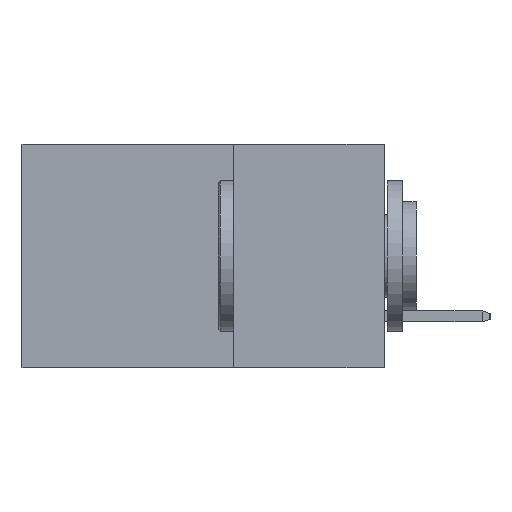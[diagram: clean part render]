
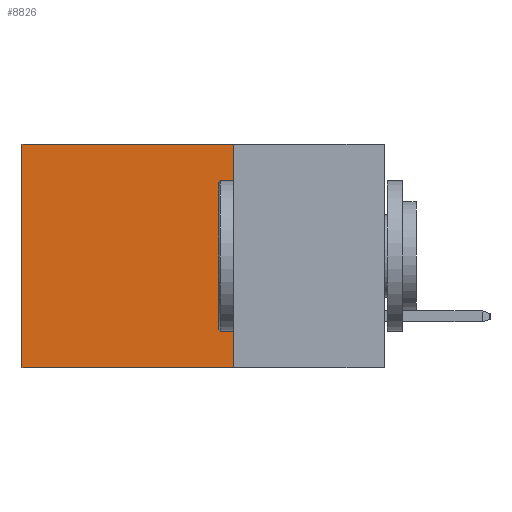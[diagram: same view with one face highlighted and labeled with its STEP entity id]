
A CAD part, left-side view. The second image highlights one B-rep face of the part: STEP entity #8826.
In plain terms, the highlighted planar face has unit normal (-1, 0, 0).
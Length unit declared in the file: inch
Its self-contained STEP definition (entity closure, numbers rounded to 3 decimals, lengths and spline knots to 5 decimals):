
#191 = DIRECTION ( 'NONE',  ( 0., 0., -1. ) ) ;
#909 = DIRECTION ( 'NONE',  ( 0., 1., 0. ) ) ;
#981 = CARTESIAN_POINT ( 'NONE',  ( 0.298, 0.25, -0.37 ) ) ;
#2281 = EDGE_CURVE ( 'NONE', #13256, #20622, #2415, .T. ) ;
#2415 = LINE ( 'NONE', #9149, #18506 ) ;
#2571 = VERTEX_POINT ( 'NONE', #17426 ) ;
#2588 = DIRECTION ( 'NONE',  ( 0., 1., 0. ) ) ;
#2706 = VECTOR ( 'NONE', #191, 39.37008 ) ;
#3196 = AXIS2_PLACEMENT_3D ( 'NONE', #12949, #9697, #21202 ) ;
#4285 = ORIENTED_EDGE ( 'NONE', *, *, #2281, .T. ) ;
#5083 = LINE ( 'NONE', #21082, #12897 ) ;
#5453 = ORIENTED_EDGE ( 'NONE', *, *, #9980, .F. ) ;
#6153 = EDGE_CURVE ( 'NONE', #2571, #19779, #18975, .T. ) ;
#6751 = CARTESIAN_POINT ( 'NONE',  ( 0.298, 0.6, 0. ) ) ;
#7078 = CARTESIAN_POINT ( 'NONE',  ( 0.298, 0.25, 0. ) ) ;
#7529 = EDGE_LOOP ( 'NONE', ( #19996, #15564, #5453, #4285 ) ) ;
#7881 = DIRECTION ( 'NONE',  ( 0., 0., -1. ) ) ;
#7948 = CARTESIAN_POINT ( 'NONE',  ( 0.298, 0.6, -0.37 ) ) ;
#8621 = CARTESIAN_POINT ( 'NONE',  ( 0.298, 0.6, 0. ) ) ;
#8826 = ADVANCED_FACE ( 'NONE', ( #9881 ), #19554, .F. ) ;
#9149 = CARTESIAN_POINT ( 'NONE',  ( 0.298, 0.25, 0. ) ) ;
#9697 = DIRECTION ( 'NONE',  ( 1., 0., 0. ) ) ;
#9881 = FACE_OUTER_BOUND ( 'NONE', #7529, .T. ) ;
#9980 = EDGE_CURVE ( 'NONE', #13256, #2571, #5083, .T. ) ;
#10270 = EDGE_CURVE ( 'NONE', #20622, #19779, #12130, .T. ) ;
#12130 = LINE ( 'NONE', #8621, #2706 ) ;
#12897 = VECTOR ( 'NONE', #7881, 39.37008 ) ;
#12949 = CARTESIAN_POINT ( 'NONE',  ( 0.298, 0.25, 0. ) ) ;
#13256 = VERTEX_POINT ( 'NONE', #7078 ) ;
#15564 = ORIENTED_EDGE ( 'NONE', *, *, #6153, .F. ) ;
#17426 = CARTESIAN_POINT ( 'NONE',  ( 0.298, 0.25, -0.37 ) ) ;
#18459 = VECTOR ( 'NONE', #909, 39.37008 ) ;
#18506 = VECTOR ( 'NONE', #2588, 39.37008 ) ;
#18975 = LINE ( 'NONE', #981, #18459 ) ;
#19554 = PLANE ( 'NONE',  #3196 ) ;
#19779 = VERTEX_POINT ( 'NONE', #7948 ) ;
#19996 = ORIENTED_EDGE ( 'NONE', *, *, #10270, .T. ) ;
#20622 = VERTEX_POINT ( 'NONE', #6751 ) ;
#21082 = CARTESIAN_POINT ( 'NONE',  ( 0.298, 0.25, 0. ) ) ;
#21202 = DIRECTION ( 'NONE',  ( 0., 0., -1. ) ) ;
